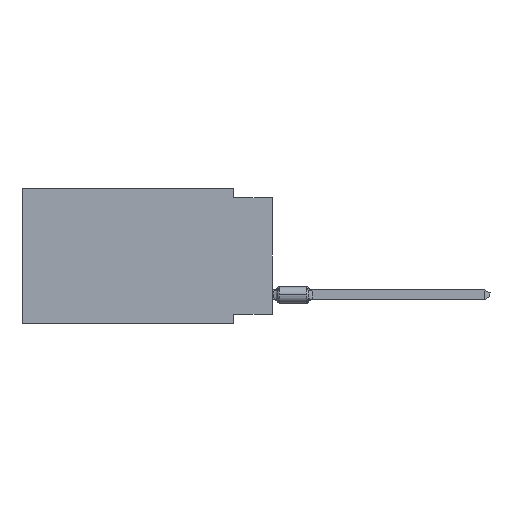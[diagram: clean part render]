
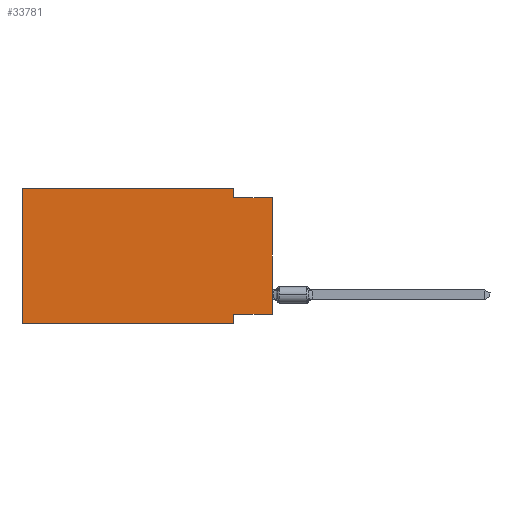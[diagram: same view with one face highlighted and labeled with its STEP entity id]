
A CAD part, left-side view. The second image highlights one B-rep face of the part: STEP entity #33781.
In plain terms, the highlighted planar face has unit normal (-1, 0, 0).
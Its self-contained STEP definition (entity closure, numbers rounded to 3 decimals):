
#600 = ORIENTED_EDGE ( 'NONE', *, *, #36457, .F. ) ;
#688 = VERTEX_POINT ( 'NONE', #43207 ) ;
#793 = CARTESIAN_POINT ( 'NONE',  ( 0., 2.54, -8.255 ) ) ;
#879 = CARTESIAN_POINT ( 'NONE',  ( 0., 0., -8.255 ) ) ;
#1880 = VERTEX_POINT ( 'NONE', #20435 ) ;
#4192 = DIRECTION ( 'NONE',  ( 0., 0., -1. ) ) ;
#4314 = ORIENTED_EDGE ( 'NONE', *, *, #10456, .F. ) ;
#4437 = PLANE ( 'NONE',  #4501 ) ;
#4501 = AXIS2_PLACEMENT_3D ( 'NONE', #43535, #23073, #4192 ) ;
#6073 = EDGE_LOOP ( 'NONE', ( #7785, #46450, #7513, #4314, #600, #19845, #21761, #20227 ) ) ;
#6288 = DIRECTION ( 'NONE',  ( 0., -1., 0. ) ) ;
#7513 = ORIENTED_EDGE ( 'NONE', *, *, #32174, .F. ) ;
#7785 = ORIENTED_EDGE ( 'NONE', *, *, #45074, .T. ) ;
#7793 = VERTEX_POINT ( 'NONE', #27532 ) ;
#10456 = EDGE_CURVE ( 'NONE', #27790, #32465, #10693, .T. ) ;
#10693 = LINE ( 'NONE', #25938, #30230 ) ;
#11614 = DIRECTION ( 'NONE',  ( 0., -1., 0. ) ) ;
#11672 = VECTOR ( 'NONE', #19790, 1000. ) ;
#12066 = VERTEX_POINT ( 'NONE', #20036 ) ;
#12287 = LINE ( 'NONE', #23645, #23129 ) ;
#12395 = VERTEX_POINT ( 'NONE', #793 ) ;
#12407 = CARTESIAN_POINT ( 'NONE',  ( 0., 2.54, 0. ) ) ;
#18268 = VERTEX_POINT ( 'NONE', #36238 ) ;
#19096 = DIRECTION ( 'NONE',  ( 0., 0., 1. ) ) ;
#19790 = DIRECTION ( 'NONE',  ( 0., 1., 0. ) ) ;
#19845 = ORIENTED_EDGE ( 'NONE', *, *, #47566, .T. ) ;
#20036 = CARTESIAN_POINT ( 'NONE',  ( 0., 0., -8.255 ) ) ;
#20227 = ORIENTED_EDGE ( 'NONE', *, *, #48859, .F. ) ;
#20435 = CARTESIAN_POINT ( 'NONE',  ( 0., 0., -0.635 ) ) ;
#21291 = LINE ( 'NONE', #25422, #26324 ) ;
#21471 = EDGE_CURVE ( 'NONE', #12395, #18268, #21291, .T. ) ;
#21761 = ORIENTED_EDGE ( 'NONE', *, *, #21471, .F. ) ;
#23008 = LINE ( 'NONE', #38793, #50898 ) ;
#23073 = DIRECTION ( 'NONE',  ( 1., 0., 0. ) ) ;
#23129 = VECTOR ( 'NONE', #28037, 1000. ) ;
#23645 = CARTESIAN_POINT ( 'NONE',  ( 0., 16.383, -8.89 ) ) ;
#23654 = LINE ( 'NONE', #879, #11672 ) ;
#24608 = EDGE_CURVE ( 'NONE', #7793, #1880, #35399, .T. ) ;
#24855 = DIRECTION ( 'NONE',  ( 0., 0., -1. ) ) ;
#25422 = CARTESIAN_POINT ( 'NONE',  ( 0., 2.54, -8.89 ) ) ;
#25938 = CARTESIAN_POINT ( 'NONE',  ( 0., 16.383, 0. ) ) ;
#26324 = VECTOR ( 'NONE', #29554, 1000. ) ;
#27532 = CARTESIAN_POINT ( 'NONE',  ( 0., 2.54, -0.635 ) ) ;
#27724 = FACE_OUTER_BOUND ( 'NONE', #6073, .T. ) ;
#27790 = VERTEX_POINT ( 'NONE', #36984 ) ;
#28037 = DIRECTION ( 'NONE',  ( 0., -1., 0. ) ) ;
#28510 = VECTOR ( 'NONE', #24855, 1000. ) ;
#29554 = DIRECTION ( 'NONE',  ( 0., 0., -1. ) ) ;
#30230 = VECTOR ( 'NONE', #6288, 1000. ) ;
#31337 = VECTOR ( 'NONE', #19096, 1000. ) ;
#32174 = EDGE_CURVE ( 'NONE', #32465, #7793, #44540, .T. ) ;
#32465 = VERTEX_POINT ( 'NONE', #12407 ) ;
#33781 = ADVANCED_FACE ( 'NONE', ( #27724 ), #4437, .F. ) ;
#35399 = LINE ( 'NONE', #51194, #35647 ) ;
#35647 = VECTOR ( 'NONE', #11614, 1000. ) ;
#36238 = CARTESIAN_POINT ( 'NONE',  ( 0., 2.54, -8.89 ) ) ;
#36457 = EDGE_CURVE ( 'NONE', #688, #27790, #23008, .T. ) ;
#36984 = CARTESIAN_POINT ( 'NONE',  ( 0., 16.383, 0. ) ) ;
#38793 = CARTESIAN_POINT ( 'NONE',  ( 0., 16.383, 0. ) ) ;
#39877 = CARTESIAN_POINT ( 'NONE',  ( 0., 2.54, 0. ) ) ;
#43207 = CARTESIAN_POINT ( 'NONE',  ( 0., 16.383, -8.89 ) ) ;
#43535 = CARTESIAN_POINT ( 'NONE',  ( 0., 16.383, 0. ) ) ;
#44540 = LINE ( 'NONE', #39877, #28510 ) ;
#45074 = EDGE_CURVE ( 'NONE', #12066, #1880, #50407, .T. ) ;
#46450 = ORIENTED_EDGE ( 'NONE', *, *, #24608, .F. ) ;
#47090 = DIRECTION ( 'NONE',  ( 0., 0., 1. ) ) ;
#47566 = EDGE_CURVE ( 'NONE', #688, #18268, #12287, .T. ) ;
#48859 = EDGE_CURVE ( 'NONE', #12066, #12395, #23654, .T. ) ;
#49894 = CARTESIAN_POINT ( 'NONE',  ( 0., 0., 0. ) ) ;
#50407 = LINE ( 'NONE', #49894, #31337 ) ;
#50898 = VECTOR ( 'NONE', #47090, 1000. ) ;
#51194 = CARTESIAN_POINT ( 'NONE',  ( 0., 0., -0.635 ) ) ;
